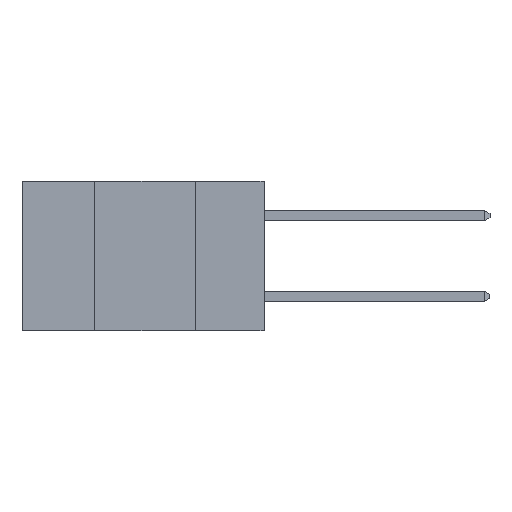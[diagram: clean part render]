
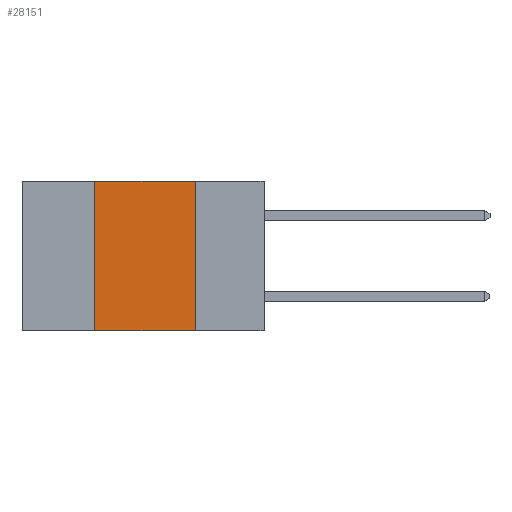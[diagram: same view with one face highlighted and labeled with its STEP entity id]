
A CAD part, left-side view. The second image highlights one B-rep face of the part: STEP entity #28151.
In plain terms, the highlighted planar face has unit normal (-1, 0, 0).
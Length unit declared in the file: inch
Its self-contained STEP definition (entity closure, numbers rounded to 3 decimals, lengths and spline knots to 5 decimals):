
#154 = ORIENTED_EDGE ( 'NONE', *, *, #23451, .F. ) ;
#612 = FACE_OUTER_BOUND ( 'NONE', #6017, .T. ) ;
#3988 = LINE ( 'NONE', #23745, #14704 ) ;
#4629 = VERTEX_POINT ( 'NONE', #7211 ) ;
#5138 = VECTOR ( 'NONE', #8549, 39.37008 ) ;
#6017 = EDGE_LOOP ( 'NONE', ( #10857, #29007, #154, #19028 ) ) ;
#6268 = CARTESIAN_POINT ( 'NONE',  ( 0., 0.6, 0. ) ) ;
#7211 = CARTESIAN_POINT ( 'NONE',  ( 0., 0.17, 0. ) ) ;
#8549 = DIRECTION ( 'NONE',  ( 0., -1., 0. ) ) ;
#10787 = CARTESIAN_POINT ( 'NONE',  ( 0., 0.17, -0.37 ) ) ;
#10857 = ORIENTED_EDGE ( 'NONE', *, *, #25000, .F. ) ;
#14564 = CARTESIAN_POINT ( 'NONE',  ( 0., 0.6, 0. ) ) ;
#14602 = CARTESIAN_POINT ( 'NONE',  ( 0., 0.42, -0.37 ) ) ;
#14663 = DIRECTION ( 'NONE',  ( 0., 0., -1. ) ) ;
#14704 = VECTOR ( 'NONE', #21570, 39.37008 ) ;
#15855 = LINE ( 'NONE', #6268, #5138 ) ;
#18755 = AXIS2_PLACEMENT_3D ( 'NONE', #14564, #28271, #14663 ) ;
#19028 = ORIENTED_EDGE ( 'NONE', *, *, #28028, .T. ) ;
#20233 = VECTOR ( 'NONE', #23323, 39.37008 ) ;
#21028 = CARTESIAN_POINT ( 'NONE',  ( 0., 0.6, -0.37 ) ) ;
#21570 = DIRECTION ( 'NONE',  ( 0., 0., -1. ) ) ;
#21659 = CARTESIAN_POINT ( 'NONE',  ( 0., 0.42, 0. ) ) ;
#23323 = DIRECTION ( 'NONE',  ( 0., -1., 0. ) ) ;
#23416 = CARTESIAN_POINT ( 'NONE',  ( 0., 0.42, 0. ) ) ;
#23451 = EDGE_CURVE ( 'NONE', #27452, #25617, #26937, .T. ) ;
#23620 = VERTEX_POINT ( 'NONE', #10787 ) ;
#23628 = EDGE_CURVE ( 'NONE', #25617, #4629, #15855, .T. ) ;
#23708 = PLANE ( 'NONE',  #18755 ) ;
#23745 = CARTESIAN_POINT ( 'NONE',  ( 0., 0.17, 0. ) ) ;
#23930 = DIRECTION ( 'NONE',  ( 0., 0., 1. ) ) ;
#24534 = LINE ( 'NONE', #21028, #20233 ) ;
#25000 = EDGE_CURVE ( 'NONE', #4629, #23620, #3988, .T. ) ;
#25617 = VERTEX_POINT ( 'NONE', #23416 ) ;
#26231 = VECTOR ( 'NONE', #23930, 39.37008 ) ;
#26937 = LINE ( 'NONE', #21659, #26231 ) ;
#27452 = VERTEX_POINT ( 'NONE', #14602 ) ;
#28028 = EDGE_CURVE ( 'NONE', #27452, #23620, #24534, .T. ) ;
#28151 = ADVANCED_FACE ( 'NONE', ( #612 ), #23708, .F. ) ;
#28271 = DIRECTION ( 'NONE',  ( 1., 0., 0. ) ) ;
#29007 = ORIENTED_EDGE ( 'NONE', *, *, #23628, .F. ) ;
